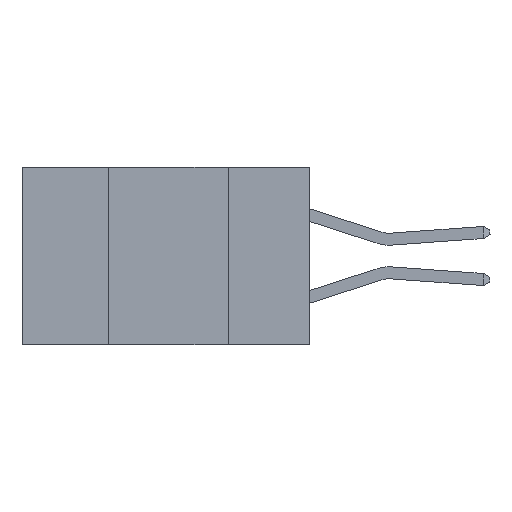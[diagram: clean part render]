
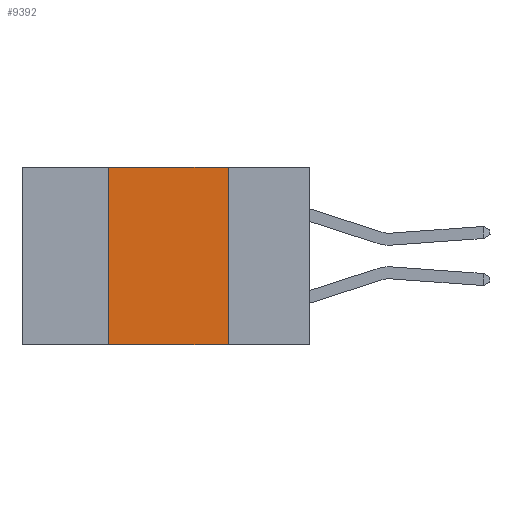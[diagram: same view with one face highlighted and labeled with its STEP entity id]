
A CAD part, left-side view. The second image highlights one B-rep face of the part: STEP entity #9392.
In plain terms, the highlighted planar face has unit normal (-1, 0, 0).
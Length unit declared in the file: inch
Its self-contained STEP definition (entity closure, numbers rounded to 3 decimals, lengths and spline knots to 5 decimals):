
#296 = VERTEX_POINT ( 'NONE', #9269 ) ;
#385 = AXIS2_PLACEMENT_3D ( 'NONE', #13845, #13760, #13724 ) ;
#778 = CARTESIAN_POINT ( 'NONE',  ( 0., 0.17, -0.37 ) ) ;
#812 = EDGE_LOOP ( 'NONE', ( #9215, #2952, #11130, #6820 ) ) ;
#921 = FACE_OUTER_BOUND ( 'NONE', #812, .T. ) ;
#1036 = DIRECTION ( 'NONE',  ( 0., 0., -1. ) ) ;
#1557 = LINE ( 'NONE', #5999, #7093 ) ;
#1995 = VECTOR ( 'NONE', #2943, 39.37008 ) ;
#2841 = LINE ( 'NONE', #5270, #11181 ) ;
#2888 = CARTESIAN_POINT ( 'NONE',  ( 0., 0.17, -0.37 ) ) ;
#2943 = DIRECTION ( 'NONE',  ( 0., 0., 1. ) ) ;
#2952 = ORIENTED_EDGE ( 'NONE', *, *, #5519, .F. ) ;
#2960 = VECTOR ( 'NONE', #1036, 39.37008 ) ;
#2974 = CARTESIAN_POINT ( 'NONE',  ( 0., 0.42, -0.37 ) ) ;
#3305 = EDGE_CURVE ( 'NONE', #7341, #4467, #2841, .T. ) ;
#4467 = VERTEX_POINT ( 'NONE', #2888 ) ;
#5151 = DIRECTION ( 'NONE',  ( 0., -1., 0. ) ) ;
#5270 = CARTESIAN_POINT ( 'NONE',  ( 0., 0.6, -0.37 ) ) ;
#5519 = EDGE_CURVE ( 'NONE', #12551, #296, #1557, .T. ) ;
#5756 = DIRECTION ( 'NONE',  ( 0., -1., 0. ) ) ;
#5999 = CARTESIAN_POINT ( 'NONE',  ( 0., 0.6, 0. ) ) ;
#6820 = ORIENTED_EDGE ( 'NONE', *, *, #3305, .T. ) ;
#7093 = VECTOR ( 'NONE', #5756, 39.37008 ) ;
#7341 = VERTEX_POINT ( 'NONE', #11592 ) ;
#8452 = EDGE_CURVE ( 'NONE', #7341, #12551, #13413, .T. ) ;
#8526 = CARTESIAN_POINT ( 'NONE',  ( 0., 0.42, 0. ) ) ;
#9215 = ORIENTED_EDGE ( 'NONE', *, *, #11975, .F. ) ;
#9269 = CARTESIAN_POINT ( 'NONE',  ( 0., 0.17, 0. ) ) ;
#9392 = ADVANCED_FACE ( 'NONE', ( #921 ), #13775, .F. ) ;
#11130 = ORIENTED_EDGE ( 'NONE', *, *, #8452, .F. ) ;
#11181 = VECTOR ( 'NONE', #5151, 39.37008 ) ;
#11592 = CARTESIAN_POINT ( 'NONE',  ( 0., 0.42, -0.37 ) ) ;
#11924 = LINE ( 'NONE', #778, #2960 ) ;
#11975 = EDGE_CURVE ( 'NONE', #296, #4467, #11924, .T. ) ;
#12551 = VERTEX_POINT ( 'NONE', #8526 ) ;
#13413 = LINE ( 'NONE', #2974, #1995 ) ;
#13724 = DIRECTION ( 'NONE',  ( 0., 0., -1. ) ) ;
#13760 = DIRECTION ( 'NONE',  ( 1., 0., 0. ) ) ;
#13775 = PLANE ( 'NONE',  #385 ) ;
#13845 = CARTESIAN_POINT ( 'NONE',  ( 0., 0.6, 0. ) ) ;
